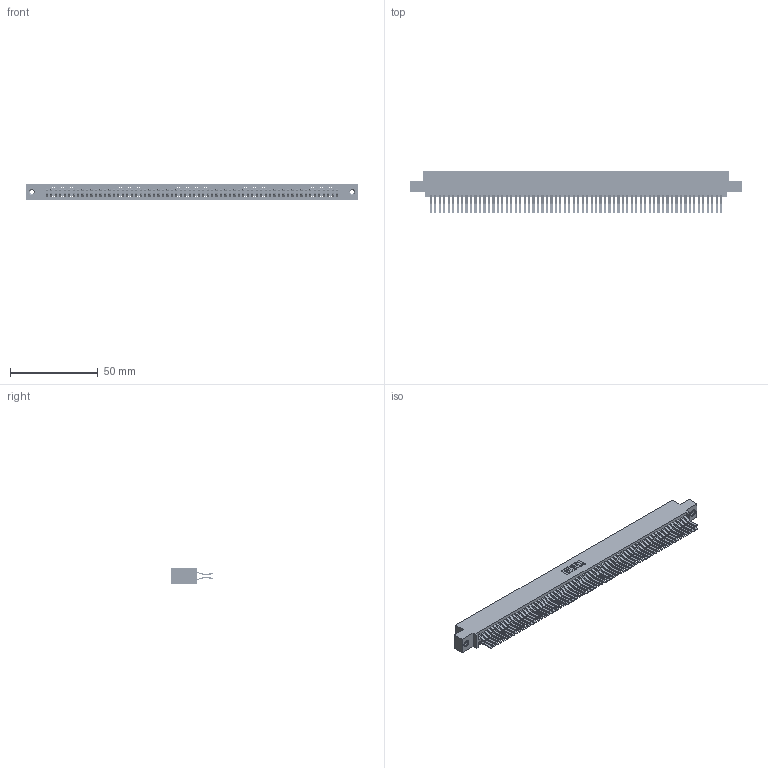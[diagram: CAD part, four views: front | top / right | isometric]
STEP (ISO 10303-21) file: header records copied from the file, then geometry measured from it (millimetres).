
FILE_DESCRIPTION (( 'STEP AP203' ), '1' );
FILE_NAME ('395-132-560-508.STEP', '2018-12-05T00:54:57', ( '' ), ( '' ), 'SwSTEP 2.0', 'SolidWorks 2016', '' );
FILE_SCHEMA (( 'CONFIG_CONTROL_DESIGN' ));
Length unit declared in the file: inch
Products named in the file (4): 395-132-560-508; 345 Part_0.110 Offset - 0.156 Dia-TI; 345-292-001_560 Tail; 345-250-001_345-250-003-102
Assembly tree (135 placements, depth 2):
  395-132-560-508
    345 Part_0.110 Offset - 0.156 Dia-TI
    345-292-001_560 Tail  x132
    345-250-001_345-250-003-102  x2
Bounding box: 188.85 x 24.45 x 9.4 mm (x, y, z)
Volume: 19353.1 mm3; surface area: 31403.4 mm2
Topology: 135 solids, 135 shells, 7054 faces, 20949 edges, 13782 vertices
Faces by surface type: plane 4472, cylinder 2566, cone 12, torus 4
Entity records: 49960 total; most frequent: CARTESIAN_POINT 8335, ORIENTED_EDGE 8262, DIRECTION 7349, EDGE_CURVE 4131, VECTOR 3711, LINE 3711, VERTEX_POINT 2748, AXIS2_PLACEMENT_3D 1819
